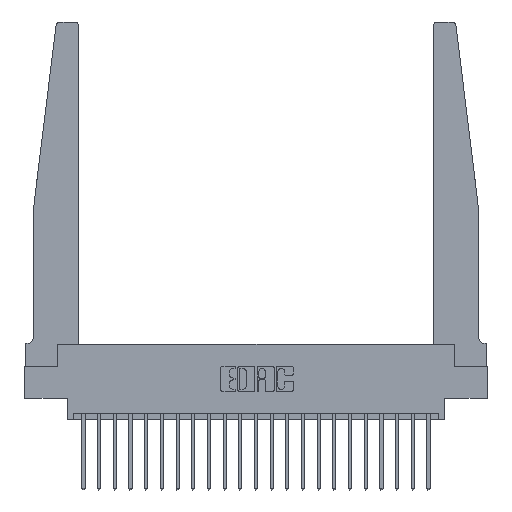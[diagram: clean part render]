
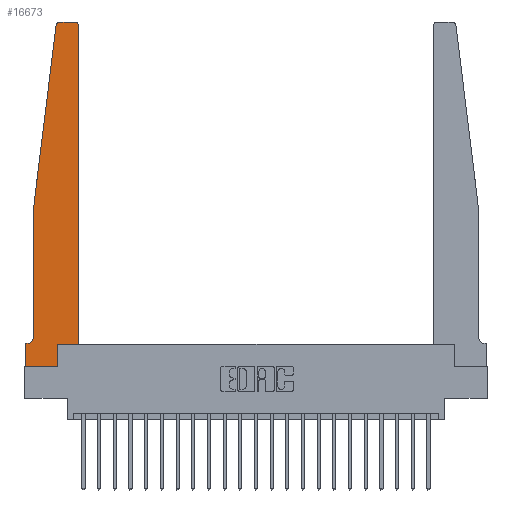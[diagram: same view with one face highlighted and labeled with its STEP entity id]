
A CAD part, top view. The second image highlights one B-rep face of the part: STEP entity #16673.
In plain terms, the highlighted planar face has unit normal (0, 0, 1).
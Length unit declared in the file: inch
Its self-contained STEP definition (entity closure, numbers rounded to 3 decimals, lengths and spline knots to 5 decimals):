
#56 = CARTESIAN_POINT ( 'NONE',  ( 0.065, 1.25, 0.37 ) ) ;
#256 = EDGE_CURVE ( 'NONE', #16925, #18684, #22732, .T. ) ;
#298 = DIRECTION ( 'NONE',  ( 1., 0., 0. ) ) ;
#408 = CARTESIAN_POINT ( 'NONE',  ( 0.065, 1.25, 0.37 ) ) ;
#537 = VERTEX_POINT ( 'NONE', #15343 ) ;
#653 = FACE_OUTER_BOUND ( 'NONE', #16469, .T. ) ;
#690 = EDGE_CURVE ( 'NONE', #11797, #12879, #20941, .T. ) ;
#947 = EDGE_CURVE ( 'NONE', #5052, #14085, #8025, .T. ) ;
#987 = CIRCLE ( 'NONE', #4680, 0.03 ) ;
#1068 = CARTESIAN_POINT ( 'NONE',  ( 0.425, 0.18, 0.37 ) ) ;
#1106 = ORIENTED_EDGE ( 'NONE', *, *, #690, .T. ) ;
#1193 = VERTEX_POINT ( 'NONE', #10986 ) ;
#1659 = CARTESIAN_POINT ( 'NONE',  ( 0.015, 0.2375, 0.37 ) ) ;
#1997 = VERTEX_POINT ( 'NONE', #8513 ) ;
#2507 = AXIS2_PLACEMENT_3D ( 'NONE', #11716, #9645, #5945 ) ;
#2622 = AXIS2_PLACEMENT_3D ( 'NONE', #12918, #4471, #5977 ) ;
#2738 = EDGE_CURVE ( 'NONE', #537, #17867, #15190, .T. ) ;
#2883 = VERTEX_POINT ( 'NONE', #21179 ) ;
#3041 = CARTESIAN_POINT ( 'NONE',  ( 0.24675, 2.72367, 0.37 ) ) ;
#3394 = EDGE_CURVE ( 'NONE', #6134, #5052, #6151, .T. ) ;
#3944 = ORIENTED_EDGE ( 'NONE', *, *, #5064, .T. ) ;
#4449 = CARTESIAN_POINT ( 'NONE',  ( 0.065, 0.1875, 0.37 ) ) ;
#4471 = DIRECTION ( 'NONE',  ( 0., 0., 1. ) ) ;
#4680 = AXIS2_PLACEMENT_3D ( 'NONE', #5621, #11173, #21646 ) ;
#5052 = VERTEX_POINT ( 'NONE', #20461 ) ;
#5064 = EDGE_CURVE ( 'NONE', #1997, #11797, #12473, .T. ) ;
#5178 = CARTESIAN_POINT ( 'NONE',  ( 0.2605, 0.18, 0.37 ) ) ;
#5621 = CARTESIAN_POINT ( 'NONE',  ( 0.395, 2.72, 0.37 ) ) ;
#5945 = DIRECTION ( 'NONE',  ( 1., 0., 0. ) ) ;
#5977 = DIRECTION ( 'NONE',  ( 1., 0., 0. ) ) ;
#6046 = DIRECTION ( 'NONE',  ( 0., 1., 0. ) ) ;
#6131 = LINE ( 'NONE', #13312, #19549 ) ;
#6134 = VERTEX_POINT ( 'NONE', #17693 ) ;
#6151 = CIRCLE ( 'NONE', #13553, 0.05 ) ;
#7096 = EDGE_CURVE ( 'NONE', #2883, #1997, #6131, .T. ) ;
#7869 = VECTOR ( 'NONE', #17290, 39.37008 ) ;
#7982 = ORIENTED_EDGE ( 'NONE', *, *, #256, .T. ) ;
#8025 = LINE ( 'NONE', #4449, #15485 ) ;
#8045 = ORIENTED_EDGE ( 'NONE', *, *, #9136, .T. ) ;
#8495 = DIRECTION ( 'NONE',  ( -1., 0., 0. ) ) ;
#8513 = CARTESIAN_POINT ( 'NONE',  ( 0.27653, 2.75, 0.37 ) ) ;
#8574 = VECTOR ( 'NONE', #21281, 39.37008 ) ;
#8795 = ORIENTED_EDGE ( 'NONE', *, *, #3394, .T. ) ;
#8984 = DIRECTION ( 'NONE',  ( 0., 1., 0. ) ) ;
#9136 = EDGE_CURVE ( 'NONE', #17867, #2883, #987, .T. ) ;
#9645 = DIRECTION ( 'NONE',  ( 0., 0., 1. ) ) ;
#9792 = CARTESIAN_POINT ( 'NONE',  ( 0., 0.1875, 0.37 ) ) ;
#10201 = CARTESIAN_POINT ( 'NONE',  ( 0., 0., 0.37 ) ) ;
#10272 = ORIENTED_EDGE ( 'NONE', *, *, #14866, .T. ) ;
#10986 = CARTESIAN_POINT ( 'NONE',  ( 0., 0., 0.37 ) ) ;
#11173 = DIRECTION ( 'NONE',  ( 0., 0., 1. ) ) ;
#11246 = CARTESIAN_POINT ( 'NONE',  ( 0.2605, 0.18, 0.37 ) ) ;
#11694 = DIRECTION ( 'NONE',  ( 1., 0., 0. ) ) ;
#11716 = CARTESIAN_POINT ( 'NONE',  ( 0.27653, 2.72, 0.37 ) ) ;
#11797 = VERTEX_POINT ( 'NONE', #3041 ) ;
#12161 = LINE ( 'NONE', #10201, #7869 ) ;
#12473 = CIRCLE ( 'NONE', #2507, 0.03 ) ;
#12742 = ORIENTED_EDGE ( 'NONE', *, *, #2738, .T. ) ;
#12811 = ORIENTED_EDGE ( 'NONE', *, *, #947, .T. ) ;
#12879 = VERTEX_POINT ( 'NONE', #13737 ) ;
#12918 = CARTESIAN_POINT ( 'NONE',  ( 0., 0.1875, 0.37 ) ) ;
#13312 = CARTESIAN_POINT ( 'NONE',  ( 0.25, 2.75, 0.37 ) ) ;
#13443 = CARTESIAN_POINT ( 'NONE',  ( 0.425, 0.18, 0.37 ) ) ;
#13553 = AXIS2_PLACEMENT_3D ( 'NONE', #1659, #21041, #8495 ) ;
#13737 = CARTESIAN_POINT ( 'NONE',  ( 0.065, 1.25, 0.37 ) ) ;
#14085 = VERTEX_POINT ( 'NONE', #9792 ) ;
#14299 = CARTESIAN_POINT ( 'NONE',  ( 0., 0., 0.37 ) ) ;
#14508 = ORIENTED_EDGE ( 'NONE', *, *, #7096, .T. ) ;
#14743 = VECTOR ( 'NONE', #15918, 39.37008 ) ;
#14866 = EDGE_CURVE ( 'NONE', #18684, #537, #17888, .T. ) ;
#15190 = LINE ( 'NONE', #1068, #20024 ) ;
#15343 = CARTESIAN_POINT ( 'NONE',  ( 0.425, 0.18, 0.37 ) ) ;
#15485 = VECTOR ( 'NONE', #16618, 39.37008 ) ;
#15918 = DIRECTION ( 'NONE',  ( -0.122, -0.992, 0. ) ) ;
#15978 = VECTOR ( 'NONE', #298, 39.37008 ) ;
#16044 = LINE ( 'NONE', #408, #8574 ) ;
#16167 = LINE ( 'NONE', #14299, #15978 ) ;
#16469 = EDGE_LOOP ( 'NONE', ( #14508, #3944, #1106, #21644, #8795, #12811, #22353, #20569, #7982, #10272, #12742, #8045 ) ) ;
#16618 = DIRECTION ( 'NONE',  ( -1., 0., 0. ) ) ;
#16673 = ADVANCED_FACE ( 'NONE', ( #653 ), #20379, .T. ) ;
#16925 = VERTEX_POINT ( 'NONE', #17786 ) ;
#17028 = DIRECTION ( 'NONE',  ( -1., 0., 0. ) ) ;
#17290 = DIRECTION ( 'NONE',  ( 0., -1., 0. ) ) ;
#17693 = CARTESIAN_POINT ( 'NONE',  ( 0.065, 0.2375, 0.37 ) ) ;
#17786 = CARTESIAN_POINT ( 'NONE',  ( 0.2605, 0., 0.37 ) ) ;
#17867 = VERTEX_POINT ( 'NONE', #18641 ) ;
#17888 = LINE ( 'NONE', #13443, #22233 ) ;
#18179 = EDGE_CURVE ( 'NONE', #12879, #6134, #16044, .T. ) ;
#18641 = CARTESIAN_POINT ( 'NONE',  ( 0.425, 2.72, 0.37 ) ) ;
#18684 = VERTEX_POINT ( 'NONE', #11246 ) ;
#18823 = VECTOR ( 'NONE', #8984, 39.37008 ) ;
#19431 = EDGE_CURVE ( 'NONE', #1193, #16925, #16167, .T. ) ;
#19549 = VECTOR ( 'NONE', #17028, 39.37008 ) ;
#20024 = VECTOR ( 'NONE', #6046, 39.37008 ) ;
#20312 = EDGE_CURVE ( 'NONE', #14085, #1193, #12161, .T. ) ;
#20379 = PLANE ( 'NONE',  #2622 ) ;
#20461 = CARTESIAN_POINT ( 'NONE',  ( 0.015, 0.1875, 0.37 ) ) ;
#20569 = ORIENTED_EDGE ( 'NONE', *, *, #19431, .T. ) ;
#20941 = LINE ( 'NONE', #56, #14743 ) ;
#21041 = DIRECTION ( 'NONE',  ( 0., 0., -1. ) ) ;
#21179 = CARTESIAN_POINT ( 'NONE',  ( 0.395, 2.75, 0.37 ) ) ;
#21281 = DIRECTION ( 'NONE',  ( 0., -1., 0. ) ) ;
#21644 = ORIENTED_EDGE ( 'NONE', *, *, #18179, .T. ) ;
#21646 = DIRECTION ( 'NONE',  ( 1., 0., 0. ) ) ;
#22233 = VECTOR ( 'NONE', #11694, 39.37008 ) ;
#22353 = ORIENTED_EDGE ( 'NONE', *, *, #20312, .T. ) ;
#22732 = LINE ( 'NONE', #5178, #18823 ) ;
